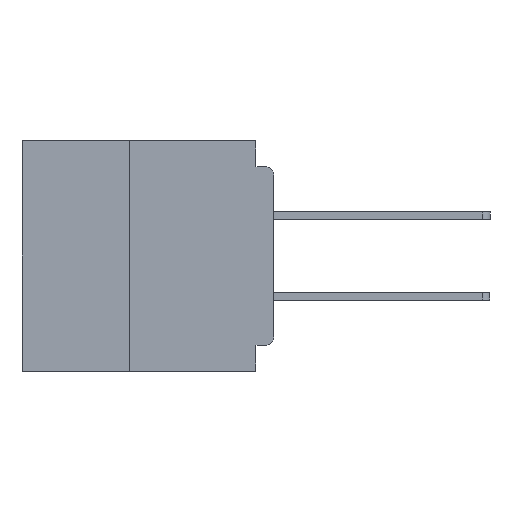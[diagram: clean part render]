
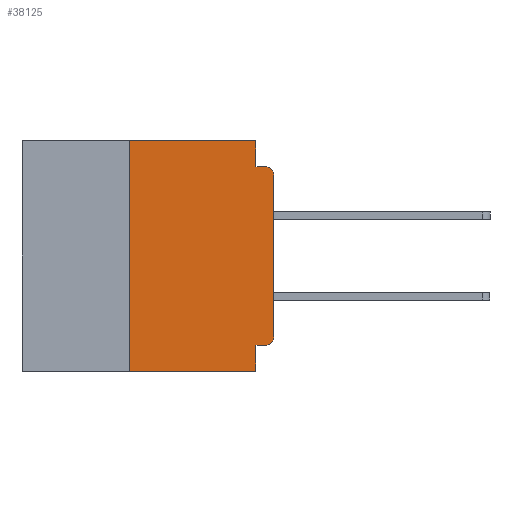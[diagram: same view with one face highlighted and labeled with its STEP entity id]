
A CAD part, left-side view. The second image highlights one B-rep face of the part: STEP entity #38125.
In plain terms, the highlighted planar face has unit normal (-1, 0, 0).
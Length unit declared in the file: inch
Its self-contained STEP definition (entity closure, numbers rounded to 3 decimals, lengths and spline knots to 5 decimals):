
#872 = EDGE_LOOP ( 'NONE', ( #38533, #32398, #14660, #40782, #19565, #31953, #14721, #12913, #13038, #9485 ) ) ;
#1295 = VERTEX_POINT ( 'NONE', #36035 ) ;
#2026 = CARTESIAN_POINT ( 'NONE',  ( 0., 0., -0.045 ) ) ;
#2850 = DIRECTION ( 'NONE',  ( 0., 0., -1. ) ) ;
#3652 = VERTEX_POINT ( 'NONE', #37032 ) ;
#4450 = CARTESIAN_POINT ( 'NONE',  ( 0., 0.437, 0. ) ) ;
#5612 = EDGE_CURVE ( 'NONE', #29815, #1295, #20353, .T. ) ;
#6433 = CARTESIAN_POINT ( 'NONE',  ( 0., 0.031, -0.4 ) ) ;
#6451 = VECTOR ( 'NONE', #21410, 39.37008 ) ;
#7466 = DIRECTION ( 'NONE',  ( -1., 0., 0. ) ) ;
#7555 = DIRECTION ( 'NONE',  ( 0., -1., 0. ) ) ;
#8116 = LINE ( 'NONE', #15585, #46307 ) ;
#8167 = DIRECTION ( 'NONE',  ( 1., 0., 0. ) ) ;
#8537 = AXIS2_PLACEMENT_3D ( 'NONE', #29637, #7466, #33330 ) ;
#9055 = VERTEX_POINT ( 'NONE', #27146 ) ;
#9485 = ORIENTED_EDGE ( 'NONE', *, *, #41049, .T. ) ;
#10134 = EDGE_CURVE ( 'NONE', #26421, #13219, #8116, .T. ) ;
#10342 = VERTEX_POINT ( 'NONE', #46546 ) ;
#10436 = VECTOR ( 'NONE', #7555, 39.37008 ) ;
#10441 = EDGE_CURVE ( 'NONE', #34830, #1295, #23793, .T. ) ;
#11780 = AXIS2_PLACEMENT_3D ( 'NONE', #41352, #19353, #45092 ) ;
#12486 = EDGE_CURVE ( 'NONE', #9055, #3652, #35712, .T. ) ;
#12729 = VECTOR ( 'NONE', #2850, 39.37008 ) ;
#12913 = ORIENTED_EDGE ( 'NONE', *, *, #10441, .F. ) ;
#13038 = ORIENTED_EDGE ( 'NONE', *, *, #36961, .F. ) ;
#13219 = VERTEX_POINT ( 'NONE', #28687 ) ;
#13792 = VECTOR ( 'NONE', #28115, 39.37008 ) ;
#14251 = CARTESIAN_POINT ( 'NONE',  ( 0., 0.25, -0.4 ) ) ;
#14660 = ORIENTED_EDGE ( 'NONE', *, *, #12486, .F. ) ;
#14721 = ORIENTED_EDGE ( 'NONE', *, *, #5612, .T. ) ;
#15176 = EDGE_CURVE ( 'NONE', #29815, #26421, #36890, .T. ) ;
#15585 = CARTESIAN_POINT ( 'NONE',  ( 0., 0.437, 0. ) ) ;
#15746 = DIRECTION ( 'NONE',  ( 0., -1., 0. ) ) ;
#16024 = CARTESIAN_POINT ( 'NONE',  ( 0., 0.031, -0.355 ) ) ;
#16350 = LINE ( 'NONE', #47057, #6451 ) ;
#18857 = VECTOR ( 'NONE', #35025, 39.37008 ) ;
#19353 = DIRECTION ( 'NONE',  ( -1., 0., 0. ) ) ;
#19565 = ORIENTED_EDGE ( 'NONE', *, *, #10134, .F. ) ;
#19740 = EDGE_CURVE ( 'NONE', #13219, #9055, #16350, .T. ) ;
#20353 = LINE ( 'NONE', #33414, #10436 ) ;
#21143 = EDGE_CURVE ( 'NONE', #26302, #3652, #45506, .T. ) ;
#21317 = AXIS2_PLACEMENT_3D ( 'NONE', #4450, #8167, #34018 ) ;
#21410 = DIRECTION ( 'NONE',  ( 0., 0., -1. ) ) ;
#22620 = EDGE_CURVE ( 'NONE', #10342, #26302, #28622, .T. ) ;
#23793 = LINE ( 'NONE', #6433, #12729 ) ;
#26302 = VERTEX_POINT ( 'NONE', #39940 ) ;
#26421 = VERTEX_POINT ( 'NONE', #33341 ) ;
#26662 = PLANE ( 'NONE',  #21317 ) ;
#27142 = VECTOR ( 'NONE', #47854, 39.37008 ) ;
#27146 = CARTESIAN_POINT ( 'NONE',  ( 0., 0.031, -0.045 ) ) ;
#28115 = DIRECTION ( 'NONE',  ( 0., -1., 0. ) ) ;
#28622 = LINE ( 'NONE', #31332, #18857 ) ;
#28687 = CARTESIAN_POINT ( 'NONE',  ( 0., 0.031, 0. ) ) ;
#29124 = CARTESIAN_POINT ( 'NONE',  ( 0., 0.25, -0.4 ) ) ;
#29637 = CARTESIAN_POINT ( 'NONE',  ( 0., 0.015, -0.06 ) ) ;
#29815 = VERTEX_POINT ( 'NONE', #29124 ) ;
#30709 = LINE ( 'NONE', #41849, #39320 ) ;
#30906 = DIRECTION ( 'NONE',  ( 0., 1., 0. ) ) ;
#31332 = CARTESIAN_POINT ( 'NONE',  ( 0., 0., 0. ) ) ;
#31344 = CARTESIAN_POINT ( 'NONE',  ( 0., 0.015, -0.355 ) ) ;
#31953 = ORIENTED_EDGE ( 'NONE', *, *, #15176, .F. ) ;
#32398 = ORIENTED_EDGE ( 'NONE', *, *, #21143, .T. ) ;
#33330 = DIRECTION ( 'NONE',  ( 0., 0., -1. ) ) ;
#33341 = CARTESIAN_POINT ( 'NONE',  ( 0., 0.25, 0. ) ) ;
#33414 = CARTESIAN_POINT ( 'NONE',  ( 0., 0.437, -0.4 ) ) ;
#34018 = DIRECTION ( 'NONE',  ( 0., 0., -1. ) ) ;
#34830 = VERTEX_POINT ( 'NONE', #16024 ) ;
#35025 = DIRECTION ( 'NONE',  ( 0., 0., 1. ) ) ;
#35712 = LINE ( 'NONE', #2026, #13792 ) ;
#36035 = CARTESIAN_POINT ( 'NONE',  ( 0., 0.031, -0.4 ) ) ;
#36890 = LINE ( 'NONE', #14251, #27142 ) ;
#36961 = EDGE_CURVE ( 'NONE', #37623, #34830, #30709, .T. ) ;
#37032 = CARTESIAN_POINT ( 'NONE',  ( 0., 0.015, -0.045 ) ) ;
#37623 = VERTEX_POINT ( 'NONE', #31344 ) ;
#38125 = ADVANCED_FACE ( 'NONE', ( #39796 ), #26662, .F. ) ;
#38533 = ORIENTED_EDGE ( 'NONE', *, *, #22620, .T. ) ;
#39320 = VECTOR ( 'NONE', #30906, 39.37008 ) ;
#39796 = FACE_OUTER_BOUND ( 'NONE', #872, .T. ) ;
#39940 = CARTESIAN_POINT ( 'NONE',  ( 0., 0., -0.06 ) ) ;
#40782 = ORIENTED_EDGE ( 'NONE', *, *, #19740, .F. ) ;
#41049 = EDGE_CURVE ( 'NONE', #37623, #10342, #45680, .T. ) ;
#41352 = CARTESIAN_POINT ( 'NONE',  ( 0., 0.015, -0.34 ) ) ;
#41849 = CARTESIAN_POINT ( 'NONE',  ( 0., 0., -0.355 ) ) ;
#45092 = DIRECTION ( 'NONE',  ( 0., 0., -1. ) ) ;
#45506 = CIRCLE ( 'NONE', #8537, 0.015 ) ;
#45680 = CIRCLE ( 'NONE', #11780, 0.015 ) ;
#46307 = VECTOR ( 'NONE', #15746, 39.37008 ) ;
#46546 = CARTESIAN_POINT ( 'NONE',  ( 0., 0., -0.34 ) ) ;
#47057 = CARTESIAN_POINT ( 'NONE',  ( 0., 0.031, 0. ) ) ;
#47854 = DIRECTION ( 'NONE',  ( 0., 0., 1. ) ) ;
